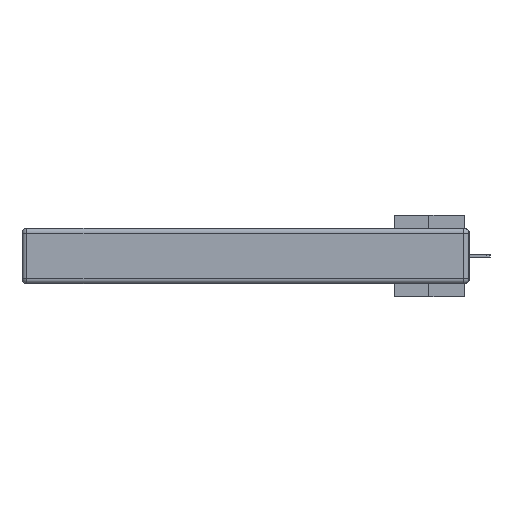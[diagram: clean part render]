
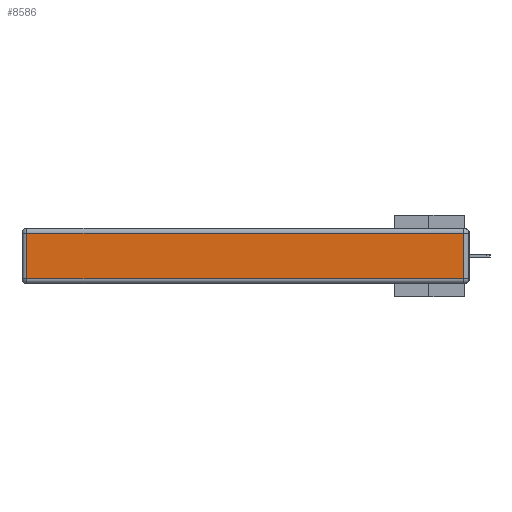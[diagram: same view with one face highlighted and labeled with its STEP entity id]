
A CAD part, left-side view. The second image highlights one B-rep face of the part: STEP entity #8586.
In plain terms, the highlighted planar face has unit normal (-1, 0, 0).
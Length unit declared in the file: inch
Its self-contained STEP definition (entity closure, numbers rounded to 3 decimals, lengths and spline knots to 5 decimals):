
#1681 = ORIENTED_EDGE ( 'NONE', *, *, #16691, .T. ) ;
#2561 = VECTOR ( 'NONE', #25310, 39.37008 ) ;
#4049 = CARTESIAN_POINT ( 'NONE',  ( 0., 2.72, -0.343 ) ) ;
#4084 = CARTESIAN_POINT ( 'NONE',  ( 0., 0.03, -0.313 ) ) ;
#4801 = CARTESIAN_POINT ( 'NONE',  ( 0., 0., -0.343 ) ) ;
#6564 = VERTEX_POINT ( 'NONE', #31846 ) ;
#6749 = LINE ( 'NONE', #4049, #30378 ) ;
#7262 = DIRECTION ( 'NONE',  ( 0., -1., 0. ) ) ;
#8136 = EDGE_LOOP ( 'NONE', ( #34051, #1681, #36052, #11453 ) ) ;
#8586 = ADVANCED_FACE ( 'NONE', ( #28121 ), #14605, .T. ) ;
#11453 = ORIENTED_EDGE ( 'NONE', *, *, #39870, .T. ) ;
#11537 = LINE ( 'NONE', #26489, #37133 ) ;
#13355 = VERTEX_POINT ( 'NONE', #4084 ) ;
#13796 = CARTESIAN_POINT ( 'NONE',  ( 0., 2.72, -0.03 ) ) ;
#14605 = PLANE ( 'NONE',  #31277 ) ;
#16223 = VECTOR ( 'NONE', #30578, 39.37008 ) ;
#16691 = EDGE_CURVE ( 'NONE', #13355, #30846, #41834, .T. ) ;
#17099 = DIRECTION ( 'NONE',  ( 0., 0., -1. ) ) ;
#17814 = DIRECTION ( 'NONE',  ( 0., 0., 1. ) ) ;
#20220 = VERTEX_POINT ( 'NONE', #13796 ) ;
#22115 = CARTESIAN_POINT ( 'NONE',  ( 0., 2.75, -0.03 ) ) ;
#22434 = CARTESIAN_POINT ( 'NONE',  ( 0., 0.03, -0.03 ) ) ;
#25310 = DIRECTION ( 'NONE',  ( 0., 1., 0. ) ) ;
#26489 = CARTESIAN_POINT ( 'NONE',  ( 0., 0., -0.313 ) ) ;
#27318 = CARTESIAN_POINT ( 'NONE',  ( 0., 0.03, -0.343 ) ) ;
#28121 = FACE_OUTER_BOUND ( 'NONE', #8136, .T. ) ;
#28359 = LINE ( 'NONE', #22115, #2561 ) ;
#28912 = EDGE_CURVE ( 'NONE', #6564, #13355, #11537, .T. ) ;
#30378 = VECTOR ( 'NONE', #17099, 39.37008 ) ;
#30578 = DIRECTION ( 'NONE',  ( 0., 0., 1. ) ) ;
#30846 = VERTEX_POINT ( 'NONE', #22434 ) ;
#31277 = AXIS2_PLACEMENT_3D ( 'NONE', #4801, #37040, #17814 ) ;
#31846 = CARTESIAN_POINT ( 'NONE',  ( 0., 2.72, -0.313 ) ) ;
#33688 = EDGE_CURVE ( 'NONE', #30846, #20220, #28359, .T. ) ;
#34051 = ORIENTED_EDGE ( 'NONE', *, *, #28912, .T. ) ;
#36052 = ORIENTED_EDGE ( 'NONE', *, *, #33688, .T. ) ;
#37040 = DIRECTION ( 'NONE',  ( -1., 0., 0. ) ) ;
#37133 = VECTOR ( 'NONE', #7262, 39.37008 ) ;
#39870 = EDGE_CURVE ( 'NONE', #20220, #6564, #6749, .T. ) ;
#41834 = LINE ( 'NONE', #27318, #16223 ) ;
